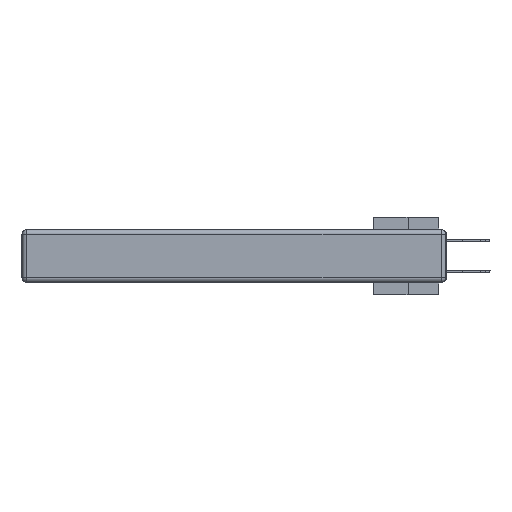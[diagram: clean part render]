
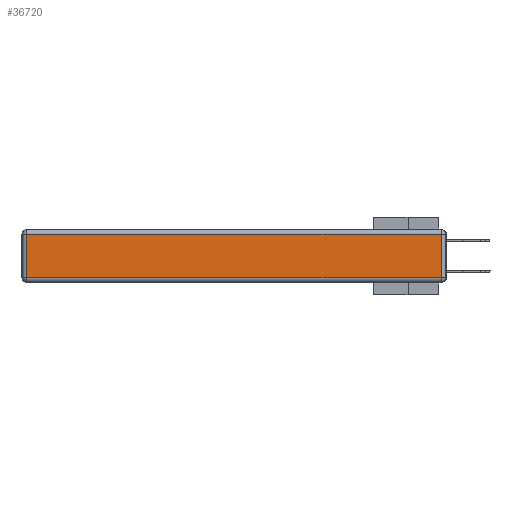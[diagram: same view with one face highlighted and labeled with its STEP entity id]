
A CAD part, left-side view. The second image highlights one B-rep face of the part: STEP entity #36720.
In plain terms, the highlighted planar face has unit normal (-1, 0, 0).
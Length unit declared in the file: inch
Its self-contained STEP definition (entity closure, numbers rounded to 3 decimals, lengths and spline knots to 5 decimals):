
#1124 = DIRECTION ( 'NONE',  ( -1., 0., 0. ) ) ;
#1302 = LINE ( 'NONE', #7995, #17121 ) ;
#2464 = VECTOR ( 'NONE', #27916, 39.37008 ) ;
#4888 = DIRECTION ( 'NONE',  ( 0., 0., -1. ) ) ;
#7995 = CARTESIAN_POINT ( 'NONE',  ( 0., 0.03, -0.343 ) ) ;
#8942 = VECTOR ( 'NONE', #4888, 39.37008 ) ;
#9378 = ORIENTED_EDGE ( 'NONE', *, *, #16787, .T. ) ;
#11508 = CARTESIAN_POINT ( 'NONE',  ( 0., 2.75, -0.03 ) ) ;
#11856 = AXIS2_PLACEMENT_3D ( 'NONE', #31476, #1124, #12544 ) ;
#12544 = DIRECTION ( 'NONE',  ( 0., 0., 1. ) ) ;
#13304 = VERTEX_POINT ( 'NONE', #25972 ) ;
#13881 = LINE ( 'NONE', #20648, #8942 ) ;
#13982 = EDGE_CURVE ( 'NONE', #24583, #15470, #20762, .T. ) ;
#15470 = VERTEX_POINT ( 'NONE', #23363 ) ;
#16787 = EDGE_CURVE ( 'NONE', #15470, #26922, #1302, .T. ) ;
#17121 = VECTOR ( 'NONE', #17694, 39.37008 ) ;
#17694 = DIRECTION ( 'NONE',  ( 0., 0., 1. ) ) ;
#20350 = CARTESIAN_POINT ( 'NONE',  ( 0., 0.03, -0.03 ) ) ;
#20648 = CARTESIAN_POINT ( 'NONE',  ( 0., 2.72, -0.343 ) ) ;
#20762 = LINE ( 'NONE', #40684, #2464 ) ;
#21964 = CARTESIAN_POINT ( 'NONE',  ( 0., 2.72, -0.313 ) ) ;
#23363 = CARTESIAN_POINT ( 'NONE',  ( 0., 0.03, -0.313 ) ) ;
#24216 = DIRECTION ( 'NONE',  ( 0., 1., 0. ) ) ;
#24583 = VERTEX_POINT ( 'NONE', #21964 ) ;
#24868 = PLANE ( 'NONE',  #11856 ) ;
#25972 = CARTESIAN_POINT ( 'NONE',  ( 0., 2.72, -0.03 ) ) ;
#26922 = VERTEX_POINT ( 'NONE', #20350 ) ;
#27916 = DIRECTION ( 'NONE',  ( 0., -1., 0. ) ) ;
#28198 = EDGE_CURVE ( 'NONE', #13304, #24583, #13881, .T. ) ;
#30320 = EDGE_LOOP ( 'NONE', ( #33975, #9378, #39522, #32347 ) ) ;
#31408 = VECTOR ( 'NONE', #24216, 39.37008 ) ;
#31476 = CARTESIAN_POINT ( 'NONE',  ( 0., 0., -0.343 ) ) ;
#32347 = ORIENTED_EDGE ( 'NONE', *, *, #28198, .T. ) ;
#33975 = ORIENTED_EDGE ( 'NONE', *, *, #13982, .T. ) ;
#35841 = EDGE_CURVE ( 'NONE', #26922, #13304, #36795, .T. ) ;
#36720 = ADVANCED_FACE ( 'NONE', ( #36756 ), #24868, .T. ) ;
#36756 = FACE_OUTER_BOUND ( 'NONE', #30320, .T. ) ;
#36795 = LINE ( 'NONE', #11508, #31408 ) ;
#39522 = ORIENTED_EDGE ( 'NONE', *, *, #35841, .T. ) ;
#40684 = CARTESIAN_POINT ( 'NONE',  ( 0., 0., -0.313 ) ) ;
